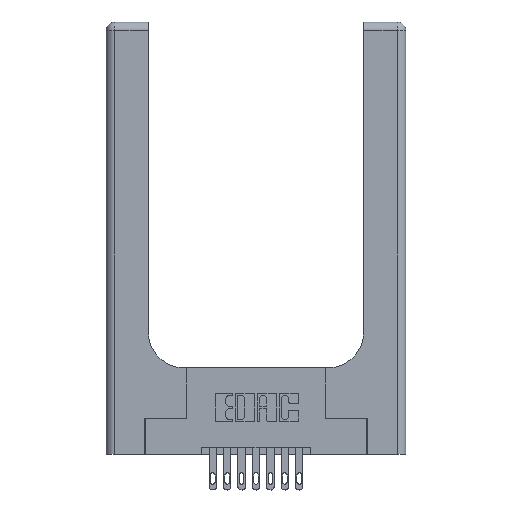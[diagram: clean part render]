
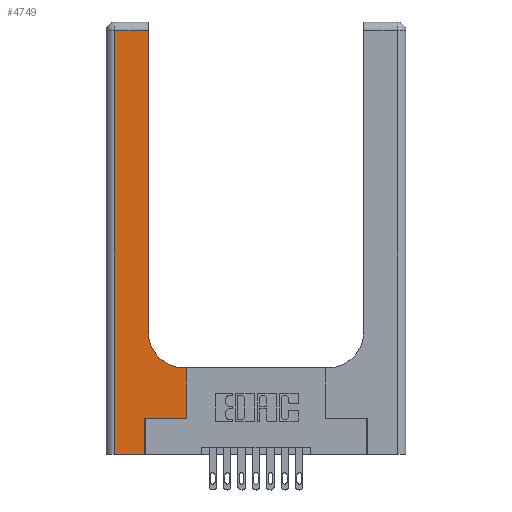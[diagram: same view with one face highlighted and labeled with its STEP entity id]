
A CAD part, top view. The second image highlights one B-rep face of the part: STEP entity #4749.
In plain terms, the highlighted planar face has unit normal (0, 0, 1).
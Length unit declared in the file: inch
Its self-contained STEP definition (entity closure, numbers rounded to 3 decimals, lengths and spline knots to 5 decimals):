
#136 = VECTOR ( 'NONE', #14579, 39.37008 ) ;
#308 = EDGE_CURVE ( 'NONE', #5778, #4908, #9355, .T. ) ;
#637 = DIRECTION ( 'NONE',  ( 0., 0., -1. ) ) ;
#689 = ORIENTED_EDGE ( 'NONE', *, *, #3983, .T. ) ;
#822 = CARTESIAN_POINT ( 'NONE',  ( 0.06, 3., 0.37 ) ) ;
#1007 = EDGE_CURVE ( 'NONE', #9794, #13108, #7675, .T. ) ;
#1195 = CARTESIAN_POINT ( 'NONE',  ( 0.5415, 0.6, 0.37 ) ) ;
#1321 = CARTESIAN_POINT ( 'NONE',  ( 0.269, 0., 0.37 ) ) ;
#1447 = EDGE_CURVE ( 'NONE', #12301, #9794, #8960, .T. ) ;
#1472 = VECTOR ( 'NONE', #13073, 39.37008 ) ;
#1489 = DIRECTION ( 'NONE',  ( -1., 0., 0. ) ) ;
#1766 = DIRECTION ( 'NONE',  ( 0., 1., 0. ) ) ;
#1777 = VECTOR ( 'NONE', #14411, 39.37008 ) ;
#1817 = CARTESIAN_POINT ( 'NONE',  ( 0.2915, 0.85, 0.37 ) ) ;
#2421 = EDGE_CURVE ( 'NONE', #7005, #7950, #15269, .T. ) ;
#2469 = CIRCLE ( 'NONE', #4654, 0.25 ) ;
#2591 = CARTESIAN_POINT ( 'NONE',  ( 0.5585, 0.25, 0.37 ) ) ;
#2737 = CARTESIAN_POINT ( 'NONE',  ( 0.2915, 0.6, 0.37 ) ) ;
#2806 = EDGE_CURVE ( 'NONE', #7950, #7929, #12644, .T. ) ;
#3161 = ORIENTED_EDGE ( 'NONE', *, *, #308, .T. ) ;
#3260 = DIRECTION ( 'NONE',  ( -1., 0., 0. ) ) ;
#3503 = EDGE_CURVE ( 'NONE', #7929, #5778, #8333, .T. ) ;
#3546 = CARTESIAN_POINT ( 'NONE',  ( 0.269, 0.25, 0.37 ) ) ;
#3895 = EDGE_LOOP ( 'NONE', ( #6637, #14277, #11042, #3161, #9360, #8203, #7161, #11467, #689 ) ) ;
#3983 = EDGE_CURVE ( 'NONE', #13108, #7005, #2469, .T. ) ;
#4145 = CARTESIAN_POINT ( 'NONE',  ( 0.2915, 3., 0.37 ) ) ;
#4231 = CARTESIAN_POINT ( 'NONE',  ( 0.5585, 0.25, 0.37 ) ) ;
#4312 = CARTESIAN_POINT ( 'NONE',  ( 0.269, 0., 0.37 ) ) ;
#4357 = DIRECTION ( 'NONE',  ( 1., 0., 0. ) ) ;
#4654 = AXIS2_PLACEMENT_3D ( 'NONE', #9008, #637, #5419 ) ;
#4749 = ADVANCED_FACE ( 'NONE', ( #6145 ), #9997, .F. ) ;
#4908 = VERTEX_POINT ( 'NONE', #1321 ) ;
#5419 = DIRECTION ( 'NONE',  ( 1., 0., 0. ) ) ;
#5778 = VERTEX_POINT ( 'NONE', #13326 ) ;
#5938 = CARTESIAN_POINT ( 'NONE',  ( 0., 0., 0.37 ) ) ;
#6145 = FACE_OUTER_BOUND ( 'NONE', #3895, .T. ) ;
#6637 = ORIENTED_EDGE ( 'NONE', *, *, #2421, .T. ) ;
#6711 = CARTESIAN_POINT ( 'NONE',  ( 0., 2.94, 0.37 ) ) ;
#7005 = VERTEX_POINT ( 'NONE', #1817 ) ;
#7161 = ORIENTED_EDGE ( 'NONE', *, *, #1447, .T. ) ;
#7646 = LINE ( 'NONE', #4312, #1777 ) ;
#7675 = LINE ( 'NONE', #2737, #10443 ) ;
#7900 = DIRECTION ( 'NONE',  ( 0., 0., -1. ) ) ;
#7929 = VERTEX_POINT ( 'NONE', #9334 ) ;
#7950 = VERTEX_POINT ( 'NONE', #8205 ) ;
#8203 = ORIENTED_EDGE ( 'NONE', *, *, #8946, .T. ) ;
#8205 = CARTESIAN_POINT ( 'NONE',  ( 0.2915, 2.94, 0.37 ) ) ;
#8333 = LINE ( 'NONE', #822, #9985 ) ;
#8346 = VECTOR ( 'NONE', #15018, 39.37008 ) ;
#8946 = EDGE_CURVE ( 'NONE', #9178, #12301, #9501, .T. ) ;
#8960 = LINE ( 'NONE', #2591, #136 ) ;
#9008 = CARTESIAN_POINT ( 'NONE',  ( 0.5415, 0.85, 0.37 ) ) ;
#9020 = EDGE_CURVE ( 'NONE', #4908, #9178, #7646, .T. ) ;
#9115 = VECTOR ( 'NONE', #1766, 39.37008 ) ;
#9143 = VECTOR ( 'NONE', #4357, 39.37008 ) ;
#9178 = VERTEX_POINT ( 'NONE', #3546 ) ;
#9334 = CARTESIAN_POINT ( 'NONE',  ( 0.06, 2.94, 0.37 ) ) ;
#9355 = LINE ( 'NONE', #5938, #1472 ) ;
#9360 = ORIENTED_EDGE ( 'NONE', *, *, #9020, .T. ) ;
#9501 = LINE ( 'NONE', #15112, #9143 ) ;
#9794 = VERTEX_POINT ( 'NONE', #10244 ) ;
#9985 = VECTOR ( 'NONE', #10219, 39.37008 ) ;
#9997 = PLANE ( 'NONE',  #13568 ) ;
#10219 = DIRECTION ( 'NONE',  ( 0., -1., 0. ) ) ;
#10244 = CARTESIAN_POINT ( 'NONE',  ( 0.5585, 0.6, 0.37 ) ) ;
#10364 = CARTESIAN_POINT ( 'NONE',  ( 0., 3., 0.37 ) ) ;
#10443 = VECTOR ( 'NONE', #1489, 39.37008 ) ;
#11042 = ORIENTED_EDGE ( 'NONE', *, *, #3503, .T. ) ;
#11467 = ORIENTED_EDGE ( 'NONE', *, *, #1007, .T. ) ;
#12301 = VERTEX_POINT ( 'NONE', #4231 ) ;
#12644 = LINE ( 'NONE', #6711, #8346 ) ;
#13073 = DIRECTION ( 'NONE',  ( 1., 0., 0. ) ) ;
#13108 = VERTEX_POINT ( 'NONE', #1195 ) ;
#13326 = CARTESIAN_POINT ( 'NONE',  ( 0.06, 0., 0.37 ) ) ;
#13568 = AXIS2_PLACEMENT_3D ( 'NONE', #10364, #7900, #3260 ) ;
#14277 = ORIENTED_EDGE ( 'NONE', *, *, #2806, .T. ) ;
#14411 = DIRECTION ( 'NONE',  ( 0., 1., 0. ) ) ;
#14579 = DIRECTION ( 'NONE',  ( 0., 1., 0. ) ) ;
#15018 = DIRECTION ( 'NONE',  ( -1., 0., 0. ) ) ;
#15112 = CARTESIAN_POINT ( 'NONE',  ( 0.269, 0.25, 0.37 ) ) ;
#15269 = LINE ( 'NONE', #4145, #9115 ) ;
